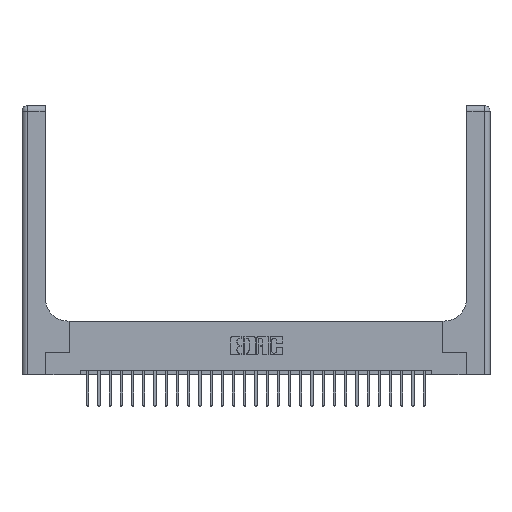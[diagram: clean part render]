
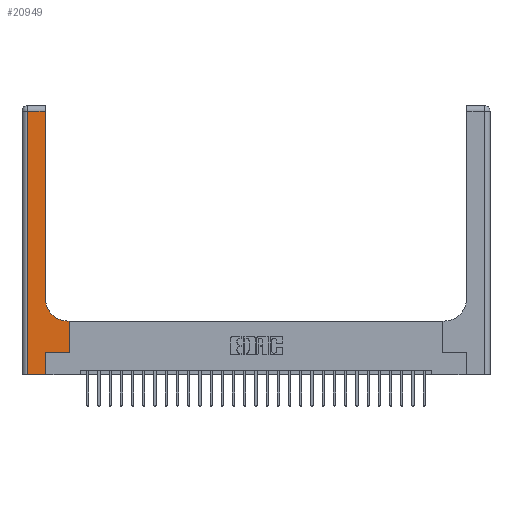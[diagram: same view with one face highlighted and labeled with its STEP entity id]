
A CAD part, top view. The second image highlights one B-rep face of the part: STEP entity #20949.
In plain terms, the highlighted planar face has unit normal (0, 0, 1).
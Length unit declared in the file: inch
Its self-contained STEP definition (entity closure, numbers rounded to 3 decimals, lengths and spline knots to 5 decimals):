
#762 = CARTESIAN_POINT ( 'NONE',  ( 0.265, 0.25, 0.37 ) ) ;
#1363 = VECTOR ( 'NONE', #9234, 39.37008 ) ;
#1619 = EDGE_LOOP ( 'NONE', ( #6758, #10495, #9793, #6715, #24524, #4496, #17140, #16407, #17247 ) ) ;
#1628 = EDGE_CURVE ( 'NONE', #18088, #3410, #24161, .T. ) ;
#2157 = VECTOR ( 'NONE', #15379, 39.37008 ) ;
#2868 = CARTESIAN_POINT ( 'NONE',  ( 0.528, 0.25, 0.37 ) ) ;
#3410 = VERTEX_POINT ( 'NONE', #19401 ) ;
#3475 = VECTOR ( 'NONE', #24254, 39.37008 ) ;
#3761 = EDGE_CURVE ( 'NONE', #20186, #18505, #15578, .T. ) ;
#3967 = DIRECTION ( 'NONE',  ( 0., 0., -1. ) ) ;
#4268 = DIRECTION ( 'NONE',  ( 1., 0., 0. ) ) ;
#4298 = LINE ( 'NONE', #26001, #13714 ) ;
#4496 = ORIENTED_EDGE ( 'NONE', *, *, #22547, .T. ) ;
#4896 = CARTESIAN_POINT ( 'NONE',  ( 0.528, 0.25, 0.37 ) ) ;
#5149 = CARTESIAN_POINT ( 'NONE',  ( 0.265, 0.25, 0.37 ) ) ;
#5257 = LINE ( 'NONE', #5149, #1363 ) ;
#5269 = LINE ( 'NONE', #5298, #21825 ) ;
#5274 = CARTESIAN_POINT ( 'NONE',  ( 0.06, 3., 0.37 ) ) ;
#5298 = CARTESIAN_POINT ( 'NONE',  ( 0.26, 3., 0.37 ) ) ;
#5586 = CARTESIAN_POINT ( 'NONE',  ( 0.265, 0., 0.37 ) ) ;
#5774 = CARTESIAN_POINT ( 'NONE',  ( 0.265, 0., 0.37 ) ) ;
#5830 = VECTOR ( 'NONE', #20385, 39.37008 ) ;
#6715 = ORIENTED_EDGE ( 'NONE', *, *, #17454, .T. ) ;
#6758 = ORIENTED_EDGE ( 'NONE', *, *, #7603, .T. ) ;
#7603 = EDGE_CURVE ( 'NONE', #23633, #8640, #5269, .T. ) ;
#7785 = CIRCLE ( 'NONE', #21844, 0.25 ) ;
#7972 = VERTEX_POINT ( 'NONE', #17495 ) ;
#8060 = EDGE_CURVE ( 'NONE', #8640, #7972, #4298, .T. ) ;
#8640 = VERTEX_POINT ( 'NONE', #15241 ) ;
#8741 = CARTESIAN_POINT ( 'NONE',  ( 0.528, 0.6, 0.37 ) ) ;
#9234 = DIRECTION ( 'NONE',  ( 1., 0., 0. ) ) ;
#9555 = DIRECTION ( 'NONE',  ( 0., 1., 0. ) ) ;
#9618 = DIRECTION ( 'NONE',  ( -1., 0., 0. ) ) ;
#9793 = ORIENTED_EDGE ( 'NONE', *, *, #11552, .T. ) ;
#10495 = ORIENTED_EDGE ( 'NONE', *, *, #8060, .T. ) ;
#11249 = VERTEX_POINT ( 'NONE', #25208 ) ;
#11552 = EDGE_CURVE ( 'NONE', #7972, #11249, #24280, .T. ) ;
#12048 = VERTEX_POINT ( 'NONE', #4896 ) ;
#12439 = CARTESIAN_POINT ( 'NONE',  ( 0., 3., 0.37 ) ) ;
#13714 = VECTOR ( 'NONE', #9618, 39.37008 ) ;
#13900 = EDGE_CURVE ( 'NONE', #12048, #18088, #16307, .T. ) ;
#14521 = LINE ( 'NONE', #17175, #2157 ) ;
#15241 = CARTESIAN_POINT ( 'NONE',  ( 0.26, 2.94, 0.37 ) ) ;
#15379 = DIRECTION ( 'NONE',  ( 1., 0., 0. ) ) ;
#15578 = LINE ( 'NONE', #5774, #5830 ) ;
#15757 = CARTESIAN_POINT ( 'NONE',  ( 0.26, 0.85, 0.37 ) ) ;
#16307 = LINE ( 'NONE', #2868, #22496 ) ;
#16407 = ORIENTED_EDGE ( 'NONE', *, *, #1628, .T. ) ;
#16498 = CARTESIAN_POINT ( 'NONE',  ( 0.51, 0.85, 0.37 ) ) ;
#17069 = AXIS2_PLACEMENT_3D ( 'NONE', #12439, #3967, #18659 ) ;
#17140 = ORIENTED_EDGE ( 'NONE', *, *, #13900, .T. ) ;
#17175 = CARTESIAN_POINT ( 'NONE',  ( 0., 0., 0.37 ) ) ;
#17247 = ORIENTED_EDGE ( 'NONE', *, *, #26185, .T. ) ;
#17454 = EDGE_CURVE ( 'NONE', #11249, #20186, #14521, .T. ) ;
#17495 = CARTESIAN_POINT ( 'NONE',  ( 0.06, 2.94, 0.37 ) ) ;
#18088 = VERTEX_POINT ( 'NONE', #8741 ) ;
#18305 = FACE_OUTER_BOUND ( 'NONE', #1619, .T. ) ;
#18471 = PLANE ( 'NONE',  #17069 ) ;
#18505 = VERTEX_POINT ( 'NONE', #762 ) ;
#18659 = DIRECTION ( 'NONE',  ( -1., 0., 0. ) ) ;
#19401 = CARTESIAN_POINT ( 'NONE',  ( 0.51, 0.6, 0.37 ) ) ;
#20186 = VERTEX_POINT ( 'NONE', #5586 ) ;
#20385 = DIRECTION ( 'NONE',  ( 0., 1., 0. ) ) ;
#20900 = VECTOR ( 'NONE', #22649, 39.37008 ) ;
#20949 = ADVANCED_FACE ( 'NONE', ( #18305 ), #18471, .F. ) ;
#21050 = DIRECTION ( 'NONE',  ( 0., 0., -1. ) ) ;
#21301 = DIRECTION ( 'NONE',  ( 0., 1., 0. ) ) ;
#21825 = VECTOR ( 'NONE', #9555, 39.37008 ) ;
#21844 = AXIS2_PLACEMENT_3D ( 'NONE', #16498, #21050, #4268 ) ;
#22496 = VECTOR ( 'NONE', #21301, 39.37008 ) ;
#22547 = EDGE_CURVE ( 'NONE', #18505, #12048, #5257, .T. ) ;
#22649 = DIRECTION ( 'NONE',  ( -1., 0., 0. ) ) ;
#23633 = VERTEX_POINT ( 'NONE', #15757 ) ;
#24161 = LINE ( 'NONE', #24946, #20900 ) ;
#24254 = DIRECTION ( 'NONE',  ( 0., -1., 0. ) ) ;
#24280 = LINE ( 'NONE', #5274, #3475 ) ;
#24524 = ORIENTED_EDGE ( 'NONE', *, *, #3761, .T. ) ;
#24946 = CARTESIAN_POINT ( 'NONE',  ( 0.26, 0.6, 0.37 ) ) ;
#25208 = CARTESIAN_POINT ( 'NONE',  ( 0.06, 0., 0.37 ) ) ;
#26001 = CARTESIAN_POINT ( 'NONE',  ( 0., 2.94, 0.37 ) ) ;
#26185 = EDGE_CURVE ( 'NONE', #3410, #23633, #7785, .T. ) ;
